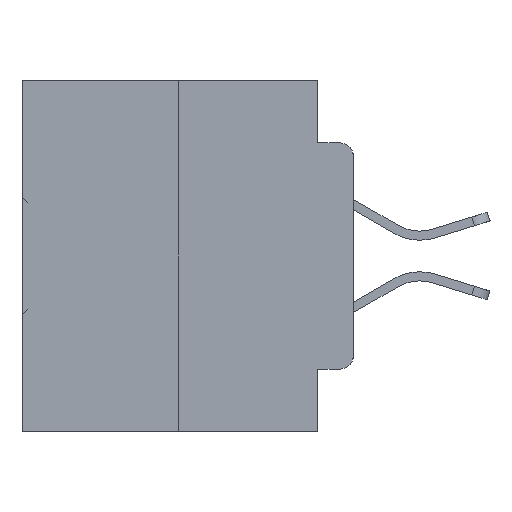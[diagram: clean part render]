
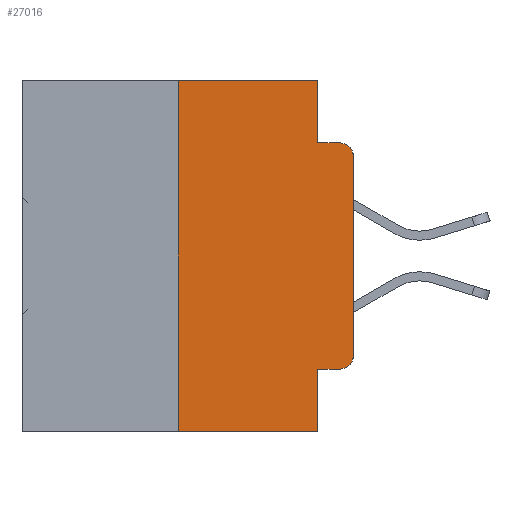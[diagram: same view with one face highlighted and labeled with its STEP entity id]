
A CAD part, left-side view. The second image highlights one B-rep face of the part: STEP entity #27016.
In plain terms, the highlighted planar face has unit normal (-1, 0, 0).
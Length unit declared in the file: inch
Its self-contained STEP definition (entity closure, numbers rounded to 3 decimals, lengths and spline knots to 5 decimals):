
#692 = AXIS2_PLACEMENT_3D ( 'NONE', #28793, #12599, #31466 ) ;
#1431 = LINE ( 'NONE', #6568, #7983 ) ;
#1503 = CIRCLE ( 'NONE', #28464, 0.02 ) ;
#1932 = DIRECTION ( 'NONE',  ( 0., 0., -1. ) ) ;
#1994 = EDGE_LOOP ( 'NONE', ( #9742, #32095, #11424, #5830, #22872, #4543, #19117, #13578, #8050, #17059 ) ) ;
#2492 = DIRECTION ( 'NONE',  ( 0., 0., -1. ) ) ;
#4235 = CARTESIAN_POINT ( 'NONE',  ( 0., 0., 0. ) ) ;
#4543 = ORIENTED_EDGE ( 'NONE', *, *, #32564, .F. ) ;
#4640 = EDGE_CURVE ( 'NONE', #7961, #28882, #8363, .T. ) ;
#4745 = VERTEX_POINT ( 'NONE', #26412 ) ;
#4783 = CARTESIAN_POINT ( 'NONE',  ( 0., 0.051, -0.0885 ) ) ;
#5212 = CARTESIAN_POINT ( 'NONE',  ( 0., 0.473, 0. ) ) ;
#5327 = EDGE_CURVE ( 'NONE', #6473, #7961, #31131, .T. ) ;
#5830 = ORIENTED_EDGE ( 'NONE', *, *, #27882, .F. ) ;
#6001 = CARTESIAN_POINT ( 'NONE',  ( 0., 0.25, 0. ) ) ;
#6473 = VERTEX_POINT ( 'NONE', #23005 ) ;
#6490 = EDGE_CURVE ( 'NONE', #27273, #10307, #15504, .T. ) ;
#6568 = CARTESIAN_POINT ( 'NONE',  ( 0., 0.25, 0. ) ) ;
#7167 = CARTESIAN_POINT ( 'NONE',  ( 0., 0.25, -0.5 ) ) ;
#7961 = VERTEX_POINT ( 'NONE', #23709 ) ;
#7983 = VECTOR ( 'NONE', #12097, 39.37008 ) ;
#8050 = ORIENTED_EDGE ( 'NONE', *, *, #18403, .T. ) ;
#8363 = CIRCLE ( 'NONE', #692, 0.02 ) ;
#9433 = VECTOR ( 'NONE', #16260, 39.37008 ) ;
#9596 = VECTOR ( 'NONE', #20633, 39.37008 ) ;
#9742 = ORIENTED_EDGE ( 'NONE', *, *, #5327, .T. ) ;
#10266 = LINE ( 'NONE', #25632, #9433 ) ;
#10307 = VERTEX_POINT ( 'NONE', #13582 ) ;
#10340 = CARTESIAN_POINT ( 'NONE',  ( 0., 0.051, -0.4115 ) ) ;
#11424 = ORIENTED_EDGE ( 'NONE', *, *, #21119, .F. ) ;
#12097 = DIRECTION ( 'NONE',  ( 0., 0., 1. ) ) ;
#12270 = LINE ( 'NONE', #30406, #32911 ) ;
#12525 = CARTESIAN_POINT ( 'NONE',  ( 0., 0.473, -0.5 ) ) ;
#12599 = DIRECTION ( 'NONE',  ( -1., 0., 0. ) ) ;
#13578 = ORIENTED_EDGE ( 'NONE', *, *, #6490, .F. ) ;
#13582 = CARTESIAN_POINT ( 'NONE',  ( 0., 0.051, -0.5 ) ) ;
#15504 = LINE ( 'NONE', #25860, #29800 ) ;
#16159 = PLANE ( 'NONE',  #27247 ) ;
#16260 = DIRECTION ( 'NONE',  ( 0., 0., -1. ) ) ;
#16878 = VECTOR ( 'NONE', #26559, 39.37008 ) ;
#17059 = ORIENTED_EDGE ( 'NONE', *, *, #29013, .T. ) ;
#17763 = EDGE_CURVE ( 'NONE', #25849, #4745, #30762, .T. ) ;
#18403 = EDGE_CURVE ( 'NONE', #27273, #19969, #31129, .T. ) ;
#18415 = DIRECTION ( 'NONE',  ( -1., 0., 0. ) ) ;
#18968 = LINE ( 'NONE', #12525, #26122 ) ;
#18975 = DIRECTION ( 'NONE',  ( 1., 0., 0. ) ) ;
#19117 = ORIENTED_EDGE ( 'NONE', *, *, #31451, .T. ) ;
#19969 = VERTEX_POINT ( 'NONE', #25064 ) ;
#20444 = DIRECTION ( 'NONE',  ( 0., 0., -1. ) ) ;
#20633 = DIRECTION ( 'NONE',  ( 0., 0., 1. ) ) ;
#21119 = EDGE_CURVE ( 'NONE', #28406, #28882, #12270, .T. ) ;
#22872 = ORIENTED_EDGE ( 'NONE', *, *, #17763, .F. ) ;
#23005 = CARTESIAN_POINT ( 'NONE',  ( 0., 0., -0.3915 ) ) ;
#23615 = VECTOR ( 'NONE', #26601, 39.37008 ) ;
#23709 = CARTESIAN_POINT ( 'NONE',  ( 0., 0., -0.1085 ) ) ;
#23895 = FACE_OUTER_BOUND ( 'NONE', #1994, .T. ) ;
#24387 = VERTEX_POINT ( 'NONE', #7167 ) ;
#25064 = CARTESIAN_POINT ( 'NONE',  ( 0., 0.02, -0.4115 ) ) ;
#25632 = CARTESIAN_POINT ( 'NONE',  ( 0., 0.051, 0. ) ) ;
#25849 = VERTEX_POINT ( 'NONE', #6001 ) ;
#25860 = CARTESIAN_POINT ( 'NONE',  ( 0., 0.051, 0. ) ) ;
#26013 = CARTESIAN_POINT ( 'NONE',  ( 0., 0.051, -0.4115 ) ) ;
#26122 = VECTOR ( 'NONE', #31381, 39.37008 ) ;
#26412 = CARTESIAN_POINT ( 'NONE',  ( 0., 0.051, 0. ) ) ;
#26559 = DIRECTION ( 'NONE',  ( 0., -1., 0. ) ) ;
#26601 = DIRECTION ( 'NONE',  ( 0., -1., 0. ) ) ;
#27016 = ADVANCED_FACE ( 'NONE', ( #23895 ), #16159, .F. ) ;
#27247 = AXIS2_PLACEMENT_3D ( 'NONE', #5212, #18975, #2492 ) ;
#27273 = VERTEX_POINT ( 'NONE', #26013 ) ;
#27882 = EDGE_CURVE ( 'NONE', #4745, #28406, #10266, .T. ) ;
#28406 = VERTEX_POINT ( 'NONE', #4783 ) ;
#28464 = AXIS2_PLACEMENT_3D ( 'NONE', #34430, #18415, #1932 ) ;
#28793 = CARTESIAN_POINT ( 'NONE',  ( 0., 0.02, -0.1085 ) ) ;
#28882 = VERTEX_POINT ( 'NONE', #33766 ) ;
#29013 = EDGE_CURVE ( 'NONE', #19969, #6473, #1503, .T. ) ;
#29304 = CARTESIAN_POINT ( 'NONE',  ( 0., 0.473, 0. ) ) ;
#29800 = VECTOR ( 'NONE', #20444, 39.37008 ) ;
#30406 = CARTESIAN_POINT ( 'NONE',  ( 0., 0.051, -0.0885 ) ) ;
#30762 = LINE ( 'NONE', #29304, #23615 ) ;
#31129 = LINE ( 'NONE', #10340, #16878 ) ;
#31131 = LINE ( 'NONE', #4235, #9596 ) ;
#31381 = DIRECTION ( 'NONE',  ( 0., -1., 0. ) ) ;
#31451 = EDGE_CURVE ( 'NONE', #24387, #10307, #18968, .T. ) ;
#31466 = DIRECTION ( 'NONE',  ( 0., 0., -1. ) ) ;
#32095 = ORIENTED_EDGE ( 'NONE', *, *, #4640, .T. ) ;
#32564 = EDGE_CURVE ( 'NONE', #24387, #25849, #1431, .T. ) ;
#32911 = VECTOR ( 'NONE', #33060, 39.37008 ) ;
#33060 = DIRECTION ( 'NONE',  ( 0., -1., 0. ) ) ;
#33766 = CARTESIAN_POINT ( 'NONE',  ( 0., 0.02, -0.0885 ) ) ;
#34430 = CARTESIAN_POINT ( 'NONE',  ( 0., 0.02, -0.3915 ) ) ;
